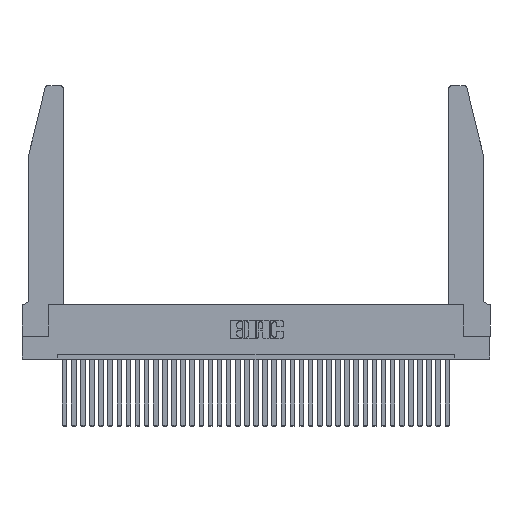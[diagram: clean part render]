
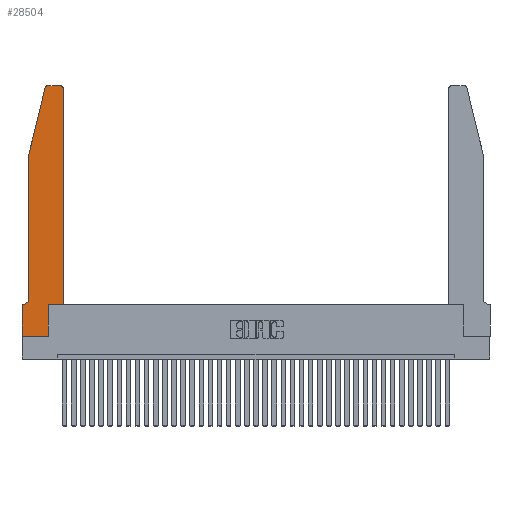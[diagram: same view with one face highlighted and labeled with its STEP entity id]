
A CAD part, top view. The second image highlights one B-rep face of the part: STEP entity #28504.
In plain terms, the highlighted planar face has unit normal (0, 0, 1).
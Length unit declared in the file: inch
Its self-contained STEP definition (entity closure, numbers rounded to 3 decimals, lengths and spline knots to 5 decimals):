
#237 = VECTOR ( 'NONE', #30913, 39.37008 ) ;
#427 = CARTESIAN_POINT ( 'NONE',  ( 0.4505, 0.35, 0.37 ) ) ;
#557 = VECTOR ( 'NONE', #15670, 39.37008 ) ;
#1898 = ORIENTED_EDGE ( 'NONE', *, *, #6629, .T. ) ;
#2195 = CIRCLE ( 'NONE', #9251, 0.03 ) ;
#2724 = DIRECTION ( 'NONE',  ( 0., 1., 0. ) ) ;
#2725 = ORIENTED_EDGE ( 'NONE', *, *, #6846, .T. ) ;
#3125 = DIRECTION ( 'NONE',  ( 0., -1., 0. ) ) ;
#3138 = DIRECTION ( 'NONE',  ( 0., 0., 1. ) ) ;
#3242 = LINE ( 'NONE', #3859, #557 ) ;
#3487 = VECTOR ( 'NONE', #5212, 39.37008 ) ;
#3680 = DIRECTION ( 'NONE',  ( -1., 0., 0. ) ) ;
#3859 = CARTESIAN_POINT ( 'NONE',  ( 0.4505, 0.35, 0.37 ) ) ;
#4296 = VERTEX_POINT ( 'NONE', #7425 ) ;
#4775 = ORIENTED_EDGE ( 'NONE', *, *, #32678, .T. ) ;
#4817 = CIRCLE ( 'NONE', #9023, 0.07 ) ;
#5054 = PLANE ( 'NONE',  #21098 ) ;
#5212 = DIRECTION ( 'NONE',  ( -1., 0., 0. ) ) ;
#5423 = VERTEX_POINT ( 'NONE', #33214 ) ;
#5931 = VERTEX_POINT ( 'NONE', #11599 ) ;
#6629 = EDGE_CURVE ( 'NONE', #8385, #25786, #3242, .T. ) ;
#6826 = CARTESIAN_POINT ( 'NONE',  ( 0.0755, 2., 0.37 ) ) ;
#6846 = EDGE_CURVE ( 'NONE', #9186, #8385, #35701, .T. ) ;
#7425 = CARTESIAN_POINT ( 'NONE',  ( 0.284, 2.75, 0.37 ) ) ;
#7615 = CARTESIAN_POINT ( 'NONE',  ( 0.4205, 2.75, 0.37 ) ) ;
#7666 = VECTOR ( 'NONE', #29788, 39.37008 ) ;
#8385 = VERTEX_POINT ( 'NONE', #18099 ) ;
#9023 = AXIS2_PLACEMENT_3D ( 'NONE', #26376, #32046, #3680 ) ;
#9186 = VERTEX_POINT ( 'NONE', #34673 ) ;
#9251 = AXIS2_PLACEMENT_3D ( 'NONE', #34081, #3138, #25595 ) ;
#9602 = DIRECTION ( 'NONE',  ( 1., 0., 0. ) ) ;
#9854 = CIRCLE ( 'NONE', #17462, 0.03 ) ;
#10131 = LINE ( 'NONE', #427, #21255 ) ;
#10226 = ORIENTED_EDGE ( 'NONE', *, *, #10899, .T. ) ;
#10464 = ORIENTED_EDGE ( 'NONE', *, *, #23239, .T. ) ;
#10803 = EDGE_CURVE ( 'NONE', #5931, #29010, #31207, .T. ) ;
#10820 = VECTOR ( 'NONE', #3125, 39.37008 ) ;
#10828 = DIRECTION ( 'NONE',  ( 1., 0., 0. ) ) ;
#10899 = EDGE_CURVE ( 'NONE', #33009, #29794, #9854, .T. ) ;
#11565 = EDGE_CURVE ( 'NONE', #29794, #4296, #25817, .T. ) ;
#11599 = CARTESIAN_POINT ( 'NONE',  ( 0.25487, 2.72718, 0.37 ) ) ;
#12522 = CARTESIAN_POINT ( 'NONE',  ( 0., 0., 0.37 ) ) ;
#13961 = DIRECTION ( 'NONE',  ( 1., 0., 0. ) ) ;
#14238 = CARTESIAN_POINT ( 'NONE',  ( 0.0755, 2., 0.37 ) ) ;
#14488 = LINE ( 'NONE', #12522, #29495 ) ;
#14853 = CARTESIAN_POINT ( 'NONE',  ( 0.0755, 2., 0.37 ) ) ;
#15670 = DIRECTION ( 'NONE',  ( 1., 0., 0. ) ) ;
#16641 = ORIENTED_EDGE ( 'NONE', *, *, #11565, .T. ) ;
#17462 = AXIS2_PLACEMENT_3D ( 'NONE', #25433, #31220, #13961 ) ;
#18099 = CARTESIAN_POINT ( 'NONE',  ( 0.2865, 0.35, 0.37 ) ) ;
#18840 = ORIENTED_EDGE ( 'NONE', *, *, #10803, .T. ) ;
#19150 = ORIENTED_EDGE ( 'NONE', *, *, #20350, .T. ) ;
#19838 = CARTESIAN_POINT ( 'NONE',  ( 0.2865, 0.35, 0.37 ) ) ;
#20291 = EDGE_LOOP ( 'NONE', ( #16641, #4775, #18840, #22073, #10464, #19150, #30041, #34394, #2725, #1898, #34587, #10226 ) ) ;
#20350 = EDGE_CURVE ( 'NONE', #30283, #31883, #34961, .T. ) ;
#20450 = EDGE_CURVE ( 'NONE', #25786, #33009, #10131, .T. ) ;
#21098 = AXIS2_PLACEMENT_3D ( 'NONE', #25215, #36293, #10828 ) ;
#21255 = VECTOR ( 'NONE', #31658, 39.37008 ) ;
#21482 = LINE ( 'NONE', #14238, #10820 ) ;
#22073 = ORIENTED_EDGE ( 'NONE', *, *, #30559, .T. ) ;
#23239 = EDGE_CURVE ( 'NONE', #5423, #30283, #4817, .T. ) ;
#23349 = EDGE_CURVE ( 'NONE', #31883, #29975, #25732, .T. ) ;
#25151 = CARTESIAN_POINT ( 'NONE',  ( 0., 0., 0.37 ) ) ;
#25215 = CARTESIAN_POINT ( 'NONE',  ( 0., 0.35, 0.37 ) ) ;
#25433 = CARTESIAN_POINT ( 'NONE',  ( 0.4205, 2.72, 0.37 ) ) ;
#25595 = DIRECTION ( 'NONE',  ( 1., 0., 0. ) ) ;
#25732 = LINE ( 'NONE', #33623, #29261 ) ;
#25786 = VERTEX_POINT ( 'NONE', #31493 ) ;
#25817 = LINE ( 'NONE', #27357, #3487 ) ;
#26223 = CARTESIAN_POINT ( 'NONE',  ( 0.0755, 0.35, 0.37 ) ) ;
#26376 = CARTESIAN_POINT ( 'NONE',  ( 0.0055, 0.42, 0.37 ) ) ;
#27188 = CARTESIAN_POINT ( 'NONE',  ( 0.4505, 2.72, 0.37 ) ) ;
#27357 = CARTESIAN_POINT ( 'NONE',  ( 0.2605, 2.75, 0.37 ) ) ;
#28504 = ADVANCED_FACE ( 'NONE', ( #32605 ), #5054, .T. ) ;
#28904 = EDGE_CURVE ( 'NONE', #29975, #9186, #14488, .T. ) ;
#29010 = VERTEX_POINT ( 'NONE', #6826 ) ;
#29261 = VECTOR ( 'NONE', #36449, 39.37008 ) ;
#29495 = VECTOR ( 'NONE', #9602, 39.37008 ) ;
#29788 = DIRECTION ( 'NONE',  ( -0.239, -0.971, 0. ) ) ;
#29794 = VERTEX_POINT ( 'NONE', #7615 ) ;
#29975 = VERTEX_POINT ( 'NONE', #25151 ) ;
#30041 = ORIENTED_EDGE ( 'NONE', *, *, #23349, .T. ) ;
#30175 = CARTESIAN_POINT ( 'NONE',  ( 0.0055, 0.35, 0.37 ) ) ;
#30283 = VERTEX_POINT ( 'NONE', #30175 ) ;
#30559 = EDGE_CURVE ( 'NONE', #29010, #5423, #21482, .T. ) ;
#30913 = DIRECTION ( 'NONE',  ( -1., 0., 0. ) ) ;
#31207 = LINE ( 'NONE', #14853, #7666 ) ;
#31220 = DIRECTION ( 'NONE',  ( 0., 0., 1. ) ) ;
#31493 = CARTESIAN_POINT ( 'NONE',  ( 0.4505, 0.35, 0.37 ) ) ;
#31658 = DIRECTION ( 'NONE',  ( 0., 1., 0. ) ) ;
#31883 = VERTEX_POINT ( 'NONE', #35463 ) ;
#32046 = DIRECTION ( 'NONE',  ( 0., 0., -1. ) ) ;
#32605 = FACE_OUTER_BOUND ( 'NONE', #20291, .T. ) ;
#32678 = EDGE_CURVE ( 'NONE', #4296, #5931, #2195, .T. ) ;
#33009 = VERTEX_POINT ( 'NONE', #27188 ) ;
#33214 = CARTESIAN_POINT ( 'NONE',  ( 0.0755, 0.42, 0.37 ) ) ;
#33623 = CARTESIAN_POINT ( 'NONE',  ( 0., 0., 0.37 ) ) ;
#34081 = CARTESIAN_POINT ( 'NONE',  ( 0.284, 2.72, 0.37 ) ) ;
#34394 = ORIENTED_EDGE ( 'NONE', *, *, #28904, .T. ) ;
#34587 = ORIENTED_EDGE ( 'NONE', *, *, #20450, .T. ) ;
#34673 = CARTESIAN_POINT ( 'NONE',  ( 0.2865, 0., 0.37 ) ) ;
#34961 = LINE ( 'NONE', #26223, #237 ) ;
#35463 = CARTESIAN_POINT ( 'NONE',  ( 0., 0.35, 0.37 ) ) ;
#35701 = LINE ( 'NONE', #19838, #36171 ) ;
#36171 = VECTOR ( 'NONE', #2724, 39.37008 ) ;
#36293 = DIRECTION ( 'NONE',  ( 0., 0., 1. ) ) ;
#36449 = DIRECTION ( 'NONE',  ( 0., -1., 0. ) ) ;
